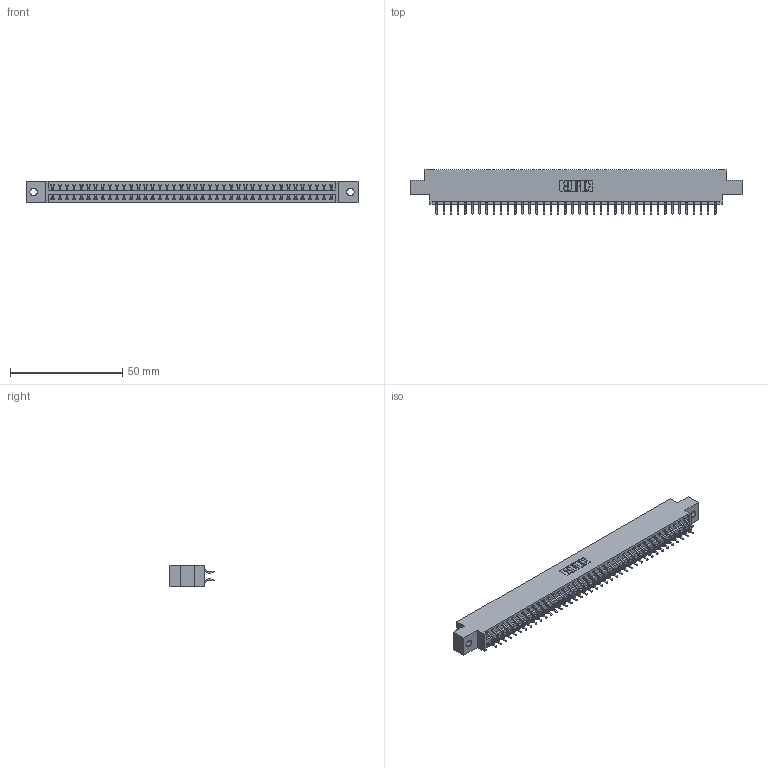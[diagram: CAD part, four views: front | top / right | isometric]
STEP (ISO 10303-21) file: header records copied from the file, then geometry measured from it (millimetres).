
FILE_DESCRIPTION (( 'STEP AP203' ), '1' );
FILE_NAME ('346-080-556-802.STEP', '2022-05-25T16:22:40', ( '' ), ( '' ), 'SwSTEP 2.0', 'SolidWorks 2020', '' );
FILE_SCHEMA (( 'CONFIG_CONTROL_DESIGN' ));
Length unit declared in the file: inch
Products named in the file (3): 346-080-556-802; 345-292-001_556 Tail; 346 Part_0.170 Offset - 0.128 Dia
Assembly tree (81 placements, depth 2):
  346-080-556-802
    346 Part_0.170 Offset - 0.128 Dia
    345-292-001_556 Tail  x80
Bounding box: 147.57 x 19.57 x 9.4 mm (x, y, z)
Volume: 14180.3 mm3; surface area: 19296.4 mm2
Topology: 81 solids, 81 shells, 4766 faces, 14181 edges, 9346 vertices
Faces by surface type: plane 3200, cylinder 1566
Entity records: 26729 total; most frequent: CARTESIAN_POINT 4424, ORIENTED_EDGE 4346, DIRECTION 3937, EDGE_CURVE 2173, LINE 1873, VECTOR 1873, VERTEX_POINT 1446, AXIS2_PLACEMENT_3D 1032
